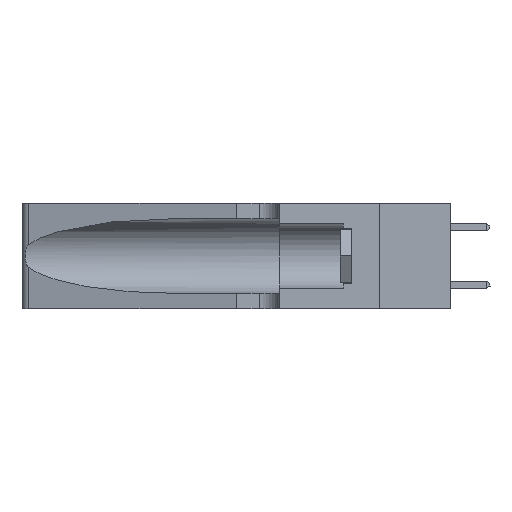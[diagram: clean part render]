
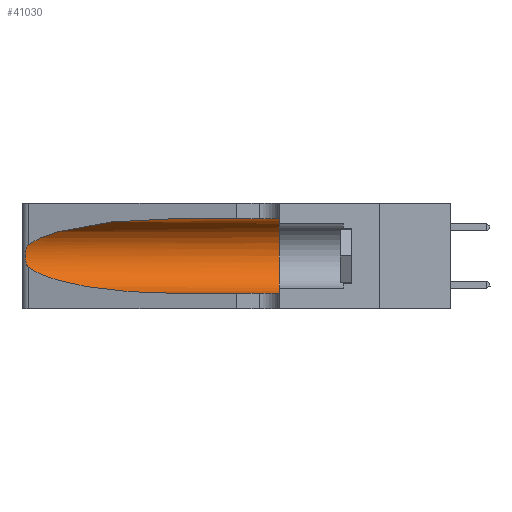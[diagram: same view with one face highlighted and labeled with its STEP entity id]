
A CAD part, left-side view. The second image highlights one B-rep face of the part: STEP entity #41030.
In plain terms, the highlighted cylindrical face has radius 3.308 mm (diameter 6.617 mm), a partial arc.
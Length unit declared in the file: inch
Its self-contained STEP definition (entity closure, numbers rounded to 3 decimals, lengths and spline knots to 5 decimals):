
#378 = AXIS2_PLACEMENT_3D ( 'NONE', #10467, #33660, #13859 ) ;
#590 = VECTOR ( 'NONE', #7609, 39.37008 ) ;
#600 = CARTESIAN_POINT ( 'NONE',  ( 0.25787, 1.23484, 0.2124 ) ) ;
#675 = VERTEX_POINT ( 'NONE', #37873 ) ;
#888 = CARTESIAN_POINT ( 'NONE',  ( 0.1305, 1.61858, 0.31525 ) ) ;
#3225 = EDGE_CURVE ( 'NONE', #35674, #26313, #14582, .T. ) ;
#3982 = CARTESIAN_POINT ( 'NONE',  ( 0.26018, 1.23835, 0.19895 ) ) ;
#4791 = ORIENTED_EDGE ( 'NONE', *, *, #6910, .F. ) ;
#5152 =( BOUNDED_CURVE ( )  B_SPLINE_CURVE ( 3, ( #18569, #38316, #11867, #41650 ),
 .UNSPECIFIED., .F., .F. ) 
 B_SPLINE_CURVE_WITH_KNOTS ( ( 4, 4 ),
 ( 3.44316, 4.71239 ),
 .UNSPECIFIED. ) 
 CURVE ( )  GEOMETRIC_REPRESENTATION_ITEM ( )  RATIONAL_B_SPLINE_CURVE ( ( 1., 0.87, 0.87, 1. ) ) 
 REPRESENTATION_ITEM ( '' )  );
#5284 = ORIENTED_EDGE ( 'NONE', *, *, #13606, .T. ) ;
#6342 = DIRECTION ( 'NONE',  ( 0., -1., 0. ) ) ;
#6910 = EDGE_CURVE ( 'NONE', #28608, #35674, #8444, .T. ) ;
#7270 = LINE ( 'NONE', #11904, #14086 ) ;
#7329 = CARTESIAN_POINT ( 'NONE',  ( 0.26075, 1.23896, 0.178 ) ) ;
#7609 = DIRECTION ( 'NONE',  ( 0., -1., 0. ) ) ;
#7698 = CARTESIAN_POINT ( 'NONE',  ( 0.25487, 1.22718, 0.14631 ) ) ;
#8444 = LINE ( 'NONE', #888, #590 ) ;
#9357 = CARTESIAN_POINT ( 'NONE',  ( 0.1305, 0.35, 0.31525 ) ) ;
#9674 =( BOUNDED_CURVE ( )  B_SPLINE_CURVE ( 3, ( #13516, #36616, #39964, #20207 ),
 .UNSPECIFIED., .F., .F. ) 
 B_SPLINE_CURVE_WITH_KNOTS ( ( 4, 4 ),
 ( 1.5708, 2.84003 ),
 .UNSPECIFIED. ) 
 CURVE ( )  GEOMETRIC_REPRESENTATION_ITEM ( )  RATIONAL_B_SPLINE_CURVE ( ( 1., 0.87, 0.87, 1. ) ) 
 REPRESENTATION_ITEM ( '' )  );
#10082 = AXIS2_PLACEMENT_3D ( 'NONE', #42697, #6342, #12962 ) ;
#10467 = CARTESIAN_POINT ( 'NONE',  ( 0.1305, 0.35, 0.185 ) ) ;
#10694 = CARTESIAN_POINT ( 'NONE',  ( 0.25856, 1.23593, 0.16098 ) ) ;
#11867 = CARTESIAN_POINT ( 'NONE',  ( 0.18966, 0.96281, 0.05475 ) ) ;
#11904 = CARTESIAN_POINT ( 'NONE',  ( 0.1305, 1.61858, 0.05475 ) ) ;
#12962 = DIRECTION ( 'NONE',  ( 0., 0., -1. ) ) ;
#13516 = CARTESIAN_POINT ( 'NONE',  ( 0.1305, 0.72297, 0.31525 ) ) ;
#13606 = EDGE_CURVE ( 'NONE', #28097, #16993, #5152, .T. ) ;
#13859 = DIRECTION ( 'NONE',  ( 0., 0., 1. ) ) ;
#14077 = CARTESIAN_POINT ( 'NONE',  ( 0.25639, 1.23186, 0.15144 ) ) ;
#14086 = VECTOR ( 'NONE', #31903, 39.37008 ) ;
#14582 = CIRCLE ( 'NONE', #378, 0.13025 ) ;
#15014 = CARTESIAN_POINT ( 'NONE',  ( 0.1305, 0.35, 0.05475 ) ) ;
#16993 = VERTEX_POINT ( 'NONE', #25271 ) ;
#17428 = CARTESIAN_POINT ( 'NONE',  ( 0.25487, 1.22718, 0.14631 ) ) ;
#18569 = CARTESIAN_POINT ( 'NONE',  ( 0.25487, 1.22718, 0.14631 ) ) ;
#19892 = ORIENTED_EDGE ( 'NONE', *, *, #38500, .T. ) ;
#20207 = CARTESIAN_POINT ( 'NONE',  ( 0.25487, 1.22718, 0.22369 ) ) ;
#20613 = CARTESIAN_POINT ( 'NONE',  ( 0.25639, 1.23184, 0.21858 ) ) ;
#23967 = CARTESIAN_POINT ( 'NONE',  ( 0.25854, 1.2359, 0.20912 ) ) ;
#24485 = FACE_OUTER_BOUND ( 'NONE', #42454, .T. ) ;
#25271 = CARTESIAN_POINT ( 'NONE',  ( 0.1305, 0.72297, 0.05475 ) ) ;
#26313 = VERTEX_POINT ( 'NONE', #15014 ) ;
#27297 = CARTESIAN_POINT ( 'NONE',  ( 0.26075, 1.23896, 0.19203 ) ) ;
#28097 = VERTEX_POINT ( 'NONE', #7698 ) ;
#28236 = ORIENTED_EDGE ( 'NONE', *, *, #3225, .F. ) ;
#28608 = VERTEX_POINT ( 'NONE', #40555 ) ;
#30608 = CARTESIAN_POINT ( 'NONE',  ( 0.26017, 1.23833, 0.17102 ) ) ;
#31807 = ORIENTED_EDGE ( 'NONE', *, *, #41550, .T. ) ;
#31903 = DIRECTION ( 'NONE',  ( 0., -1., 0. ) ) ;
#33660 = DIRECTION ( 'NONE',  ( 0., 1., 0. ) ) ;
#33873 = CARTESIAN_POINT ( 'NONE',  ( 0.25789, 1.23486, 0.15765 ) ) ;
#35144 = EDGE_CURVE ( 'NONE', #28608, #675, #9674, .T. ) ;
#35674 = VERTEX_POINT ( 'NONE', #9357 ) ;
#36374 = ORIENTED_EDGE ( 'NONE', *, *, #35144, .T. ) ;
#36616 = CARTESIAN_POINT ( 'NONE',  ( 0.18966, 0.96281, 0.31525 ) ) ;
#37022 = CARTESIAN_POINT ( 'NONE',  ( 0.25487, 1.22718, 0.22369 ) ) ;
#37169 = CARTESIAN_POINT ( 'NONE',  ( 0.25555, 1.22993, 0.14849 ) ) ;
#37284 = B_SPLINE_CURVE_WITH_KNOTS ( 'NONE', 3,
 ( #37022, #40364, #20613, #600, #23967, #3982, #27297, #7329, #30608, #10694, #33873, #14077, #37169, #17428 ),
 .UNSPECIFIED., .F., .F.,
 ( 4, 2, 2, 2, 2, 2, 4 ),
 ( 0., 0.00027, 0.00053, 0.00107, 0.0016, 0.00187, 0.00214 ),
 .UNSPECIFIED. ) ;
#37873 = CARTESIAN_POINT ( 'NONE',  ( 0.25487, 1.22718, 0.22369 ) ) ;
#38316 = CARTESIAN_POINT ( 'NONE',  ( 0.2373, 1.15595, 0.08982 ) ) ;
#38500 = EDGE_CURVE ( 'NONE', #675, #28097, #37284, .T. ) ;
#39964 = CARTESIAN_POINT ( 'NONE',  ( 0.2373, 1.15595, 0.28018 ) ) ;
#40364 = CARTESIAN_POINT ( 'NONE',  ( 0.25555, 1.22994, 0.2215 ) ) ;
#40555 = CARTESIAN_POINT ( 'NONE',  ( 0.1305, 0.72297, 0.31525 ) ) ;
#40946 = CYLINDRICAL_SURFACE ( 'NONE', #10082, 0.13025 ) ;
#41030 = ADVANCED_FACE ( 'NONE', ( #24485 ), #40946, .F. ) ;
#41550 = EDGE_CURVE ( 'NONE', #16993, #26313, #7270, .T. ) ;
#41650 = CARTESIAN_POINT ( 'NONE',  ( 0.1305, 0.72297, 0.05475 ) ) ;
#42454 = EDGE_LOOP ( 'NONE', ( #36374, #19892, #5284, #31807, #28236, #4791 ) ) ;
#42697 = CARTESIAN_POINT ( 'NONE',  ( 0.1305, 1.61858, 0.185 ) ) ;
